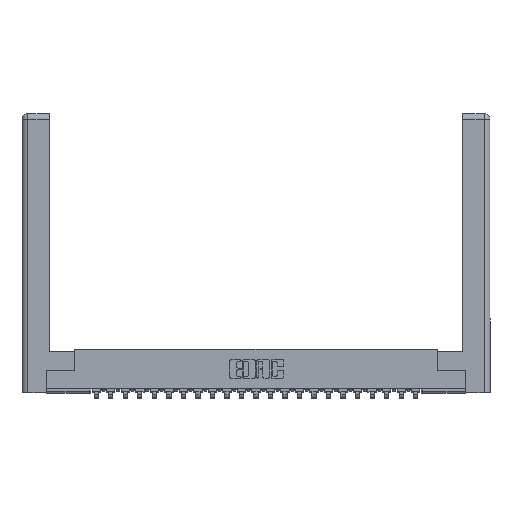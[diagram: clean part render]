
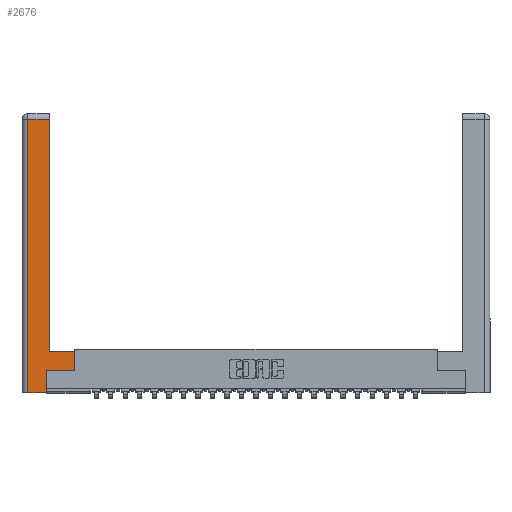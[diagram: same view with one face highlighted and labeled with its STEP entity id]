
A CAD part, top view. The second image highlights one B-rep face of the part: STEP entity #2676.
In plain terms, the highlighted planar face has unit normal (0, 0, 1).
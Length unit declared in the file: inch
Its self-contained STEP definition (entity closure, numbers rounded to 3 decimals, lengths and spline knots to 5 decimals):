
#889 = LINE ( 'NONE', #6936, #2563 ) ;
#1047 = VECTOR ( 'NONE', #1196, 39.37008 ) ;
#1196 = DIRECTION ( 'NONE',  ( -1., 0., 0. ) ) ;
#1199 = VECTOR ( 'NONE', #13073, 39.37008 ) ;
#1381 = VERTEX_POINT ( 'NONE', #2744 ) ;
#2563 = VECTOR ( 'NONE', #4631, 39.37008 ) ;
#2664 = DIRECTION ( 'NONE',  ( -1., 0., 0. ) ) ;
#2676 = ADVANCED_FACE ( 'NONE', ( #18186 ), #2939, .F. ) ;
#2744 = CARTESIAN_POINT ( 'NONE',  ( 0.265, 0.245, 0. ) ) ;
#2792 = VECTOR ( 'NONE', #13567, 39.37008 ) ;
#2939 = PLANE ( 'NONE',  #14611 ) ;
#3273 = LINE ( 'NONE', #4812, #18142 ) ;
#4457 = CARTESIAN_POINT ( 'NONE',  ( 0.0615, 0., 0. ) ) ;
#4631 = DIRECTION ( 'NONE',  ( 0., -1., 0. ) ) ;
#4812 = CARTESIAN_POINT ( 'NONE',  ( 0.565, 0.45, 0. ) ) ;
#5016 = CARTESIAN_POINT ( 'NONE',  ( 0.565, 0.45, 0. ) ) ;
#5681 = ORIENTED_EDGE ( 'NONE', *, *, #9139, .T. ) ;
#5854 = VECTOR ( 'NONE', #23803, 39.37008 ) ;
#6185 = CARTESIAN_POINT ( 'NONE',  ( 0.0615, 2.94, 0. ) ) ;
#6277 = LINE ( 'NONE', #16108, #6951 ) ;
#6304 = CARTESIAN_POINT ( 'NONE',  ( 0.265, 0., 0. ) ) ;
#6405 = DIRECTION ( 'NONE',  ( 1., 0., 0. ) ) ;
#6936 = CARTESIAN_POINT ( 'NONE',  ( 0.0615, 0., 0. ) ) ;
#6951 = VECTOR ( 'NONE', #6405, 39.37008 ) ;
#7323 = VERTEX_POINT ( 'NONE', #4457 ) ;
#7862 = VECTOR ( 'NONE', #2664, 39.37008 ) ;
#8255 = LINE ( 'NONE', #21972, #5854 ) ;
#8835 = ORIENTED_EDGE ( 'NONE', *, *, #23152, .T. ) ;
#8871 = ORIENTED_EDGE ( 'NONE', *, *, #25239, .T. ) ;
#9139 = EDGE_CURVE ( 'NONE', #13025, #14215, #9192, .T. ) ;
#9192 = LINE ( 'NONE', #24979, #1047 ) ;
#9706 = ORIENTED_EDGE ( 'NONE', *, *, #13901, .T. ) ;
#10114 = CARTESIAN_POINT ( 'NONE',  ( 0.295, 0.45, 0. ) ) ;
#10426 = VERTEX_POINT ( 'NONE', #6185 ) ;
#10646 = LINE ( 'NONE', #18553, #7862 ) ;
#10853 = ORIENTED_EDGE ( 'NONE', *, *, #19169, .T. ) ;
#11594 = VERTEX_POINT ( 'NONE', #19668 ) ;
#11630 = LINE ( 'NONE', #21470, #2792 ) ;
#12080 = VERTEX_POINT ( 'NONE', #15850 ) ;
#12957 = DIRECTION ( 'NONE',  ( 0., 1., 0. ) ) ;
#13025 = VERTEX_POINT ( 'NONE', #5016 ) ;
#13073 = DIRECTION ( 'NONE',  ( 0., 1., 0. ) ) ;
#13567 = DIRECTION ( 'NONE',  ( 0., 1., 0. ) ) ;
#13901 = EDGE_CURVE ( 'NONE', #12080, #10426, #10646, .T. ) ;
#14215 = VERTEX_POINT ( 'NONE', #10114 ) ;
#14611 = AXIS2_PLACEMENT_3D ( 'NONE', #18706, #18319, #22347 ) ;
#15508 = LINE ( 'NONE', #16935, #1199 ) ;
#15850 = CARTESIAN_POINT ( 'NONE',  ( 0.295, 2.94, 0. ) ) ;
#15874 = EDGE_LOOP ( 'NONE', ( #10853, #9706, #8871, #16577, #22127, #21920, #8835, #5681 ) ) ;
#16108 = CARTESIAN_POINT ( 'NONE',  ( 0.565, 0.245, 0. ) ) ;
#16577 = ORIENTED_EDGE ( 'NONE', *, *, #25111, .T. ) ;
#16935 = CARTESIAN_POINT ( 'NONE',  ( 0.265, 0.245, 0. ) ) ;
#18142 = VECTOR ( 'NONE', #12957, 39.37008 ) ;
#18186 = FACE_OUTER_BOUND ( 'NONE', #15874, .T. ) ;
#18319 = DIRECTION ( 'NONE',  ( 0., 0., -1. ) ) ;
#18354 = VERTEX_POINT ( 'NONE', #6304 ) ;
#18553 = CARTESIAN_POINT ( 'NONE',  ( 0.0615, 2.94, 0. ) ) ;
#18706 = CARTESIAN_POINT ( 'NONE',  ( 0., 0., 0. ) ) ;
#19169 = EDGE_CURVE ( 'NONE', #14215, #12080, #11630, .T. ) ;
#19668 = CARTESIAN_POINT ( 'NONE',  ( 0.565, 0.245, 0. ) ) ;
#20942 = EDGE_CURVE ( 'NONE', #1381, #11594, #6277, .T. ) ;
#21470 = CARTESIAN_POINT ( 'NONE',  ( 0.295, 3., 0. ) ) ;
#21920 = ORIENTED_EDGE ( 'NONE', *, *, #20942, .T. ) ;
#21972 = CARTESIAN_POINT ( 'NONE',  ( 0.265, 0., 0. ) ) ;
#22127 = ORIENTED_EDGE ( 'NONE', *, *, #22212, .T. ) ;
#22212 = EDGE_CURVE ( 'NONE', #18354, #1381, #15508, .T. ) ;
#22347 = DIRECTION ( 'NONE',  ( -1., 0., 0. ) ) ;
#23152 = EDGE_CURVE ( 'NONE', #11594, #13025, #3273, .T. ) ;
#23803 = DIRECTION ( 'NONE',  ( 1., 0., 0. ) ) ;
#24979 = CARTESIAN_POINT ( 'NONE',  ( 0.295, 0.45, 0. ) ) ;
#25111 = EDGE_CURVE ( 'NONE', #7323, #18354, #8255, .T. ) ;
#25239 = EDGE_CURVE ( 'NONE', #10426, #7323, #889, .T. ) ;
